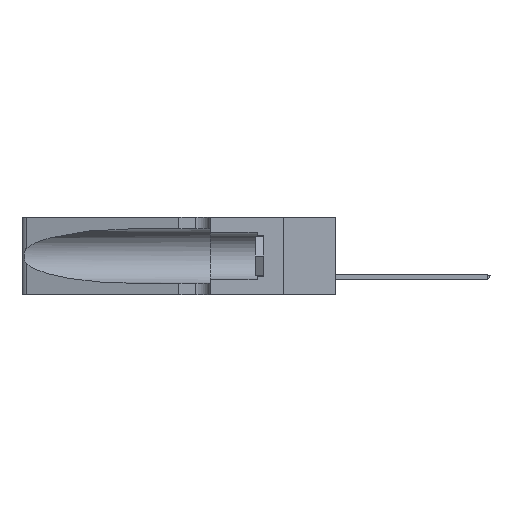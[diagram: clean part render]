
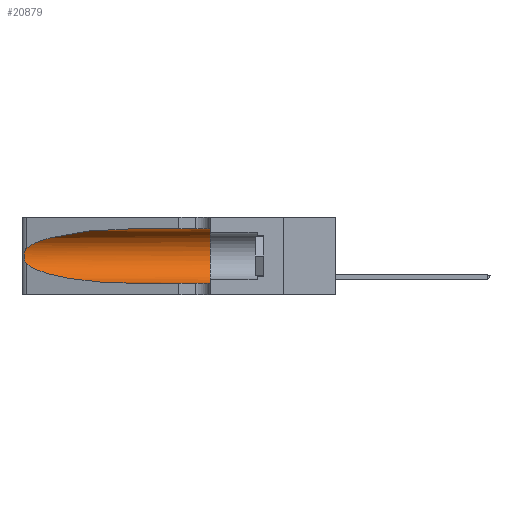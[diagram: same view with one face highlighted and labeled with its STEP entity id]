
A CAD part, left-side view. The second image highlights one B-rep face of the part: STEP entity #20879.
In plain terms, the highlighted cylindrical face has radius 3.308 mm (diameter 6.617 mm), a partial arc.
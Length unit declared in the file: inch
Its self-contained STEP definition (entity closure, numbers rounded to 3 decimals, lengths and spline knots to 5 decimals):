
#116 = B_SPLINE_CURVE_WITH_KNOTS ( 'NONE', 3,
 ( #9025, #15880, #19673, #1629, #12503, #10636, #21319, #10792, #19597, #17581, #23099, #5159, #19377, #5382 ),
 .UNSPECIFIED., .F., .F.,
 ( 4, 2, 2, 2, 2, 2, 4 ),
 ( 0., 0.00027, 0.00053, 0.00107, 0.0016, 0.00187, 0.00214 ),
 .UNSPECIFIED. ) ;
#762 = ORIENTED_EDGE ( 'NONE', *, *, #16962, .F. ) ;
#1184 = ORIENTED_EDGE ( 'NONE', *, *, #10674, .T. ) ;
#1629 = CARTESIAN_POINT ( 'NONE',  ( 0.25787, 1.23484, 0.2124 ) ) ;
#1871 = EDGE_CURVE ( 'NONE', #15046, #11909, #20135, .T. ) ;
#1888 = AXIS2_PLACEMENT_3D ( 'NONE', #19101, #22509, #6600 ) ;
#1976 = EDGE_CURVE ( 'NONE', #8461, #4619, #5324, .T. ) ;
#3780 = ORIENTED_EDGE ( 'NONE', *, *, #1871, .T. ) ;
#3968 = CARTESIAN_POINT ( 'NONE',  ( 0.18966, 0.96281, 0.31525 ) ) ;
#4028 = CYLINDRICAL_SURFACE ( 'NONE', #13454, 0.13025 ) ;
#4334 = LINE ( 'NONE', #12100, #22416 ) ;
#4619 = VERTEX_POINT ( 'NONE', #10180 ) ;
#5159 = CARTESIAN_POINT ( 'NONE',  ( 0.25639, 1.23186, 0.15144 ) ) ;
#5324 =( BOUNDED_CURVE ( )  B_SPLINE_CURVE ( 3, ( #9031, #3968, #19676, #19816 ),
 .UNSPECIFIED., .F., .T. ) 
 B_SPLINE_CURVE_WITH_KNOTS ( ( 4, 4 ),
 ( 1.5708, 2.84003 ),
 .UNSPECIFIED. ) 
 CURVE ( )  GEOMETRIC_REPRESENTATION_ITEM ( )  RATIONAL_B_SPLINE_CURVE ( ( 1., 0.87, 0.87, 1. ) ) 
 REPRESENTATION_ITEM ( '' )  );
#5382 = CARTESIAN_POINT ( 'NONE',  ( 0.25487, 1.22718, 0.14631 ) ) ;
#6600 = DIRECTION ( 'NONE',  ( 0., 0., 1. ) ) ;
#7967 = CIRCLE ( 'NONE', #1888, 0.13025 ) ;
#8461 = VERTEX_POINT ( 'NONE', #8618 ) ;
#8618 = CARTESIAN_POINT ( 'NONE',  ( 0.1305, 0.72297, 0.31525 ) ) ;
#8760 = FACE_OUTER_BOUND ( 'NONE', #20014, .T. ) ;
#8932 = CARTESIAN_POINT ( 'NONE',  ( 0.1305, 0.72297, 0.05475 ) ) ;
#9025 = CARTESIAN_POINT ( 'NONE',  ( 0.25487, 1.22718, 0.22369 ) ) ;
#9031 = CARTESIAN_POINT ( 'NONE',  ( 0.1305, 0.72297, 0.31525 ) ) ;
#9729 = DIRECTION ( 'NONE',  ( 0., -1., 0. ) ) ;
#10069 = ORIENTED_EDGE ( 'NONE', *, *, #19679, .F. ) ;
#10180 = CARTESIAN_POINT ( 'NONE',  ( 0.25487, 1.22718, 0.22369 ) ) ;
#10636 = CARTESIAN_POINT ( 'NONE',  ( 0.26018, 1.23835, 0.19895 ) ) ;
#10674 = EDGE_CURVE ( 'NONE', #11909, #17735, #15838, .T. ) ;
#10792 = CARTESIAN_POINT ( 'NONE',  ( 0.26075, 1.23896, 0.178 ) ) ;
#11480 = DIRECTION ( 'NONE',  ( 0., 0., -1. ) ) ;
#11909 = VERTEX_POINT ( 'NONE', #8932 ) ;
#12100 = CARTESIAN_POINT ( 'NONE',  ( 0.1305, 1.61858, 0.31525 ) ) ;
#12145 = CARTESIAN_POINT ( 'NONE',  ( 0.1305, 1.61858, 0.05475 ) ) ;
#12161 = ORIENTED_EDGE ( 'NONE', *, *, #13159, .T. ) ;
#12503 = CARTESIAN_POINT ( 'NONE',  ( 0.25854, 1.2359, 0.20912 ) ) ;
#13159 = EDGE_CURVE ( 'NONE', #4619, #15046, #116, .T. ) ;
#13454 = AXIS2_PLACEMENT_3D ( 'NONE', #15027, #9729, #11480 ) ;
#14112 = CARTESIAN_POINT ( 'NONE',  ( 0.25487, 1.22718, 0.14631 ) ) ;
#14840 = CARTESIAN_POINT ( 'NONE',  ( 0.25487, 1.22718, 0.14631 ) ) ;
#15011 = CARTESIAN_POINT ( 'NONE',  ( 0.1305, 0.35, 0.05475 ) ) ;
#15027 = CARTESIAN_POINT ( 'NONE',  ( 0.1305, 1.61858, 0.185 ) ) ;
#15046 = VERTEX_POINT ( 'NONE', #14112 ) ;
#15838 = LINE ( 'NONE', #12145, #20541 ) ;
#15852 = DIRECTION ( 'NONE',  ( 0., -1., 0. ) ) ;
#15880 = CARTESIAN_POINT ( 'NONE',  ( 0.25555, 1.22994, 0.2215 ) ) ;
#16962 = EDGE_CURVE ( 'NONE', #19148, #17735, #7967, .T. ) ;
#17161 = CARTESIAN_POINT ( 'NONE',  ( 0.2373, 1.15595, 0.08982 ) ) ;
#17473 = CARTESIAN_POINT ( 'NONE',  ( 0.1305, 0.72297, 0.05475 ) ) ;
#17581 = CARTESIAN_POINT ( 'NONE',  ( 0.25856, 1.23593, 0.16098 ) ) ;
#17735 = VERTEX_POINT ( 'NONE', #15011 ) ;
#19101 = CARTESIAN_POINT ( 'NONE',  ( 0.1305, 0.35, 0.185 ) ) ;
#19148 = VERTEX_POINT ( 'NONE', #19623 ) ;
#19377 = CARTESIAN_POINT ( 'NONE',  ( 0.25555, 1.22993, 0.14849 ) ) ;
#19597 = CARTESIAN_POINT ( 'NONE',  ( 0.26017, 1.23833, 0.17102 ) ) ;
#19623 = CARTESIAN_POINT ( 'NONE',  ( 0.1305, 0.35, 0.31525 ) ) ;
#19673 = CARTESIAN_POINT ( 'NONE',  ( 0.25639, 1.23184, 0.21858 ) ) ;
#19676 = CARTESIAN_POINT ( 'NONE',  ( 0.2373, 1.15595, 0.28018 ) ) ;
#19679 = EDGE_CURVE ( 'NONE', #8461, #19148, #4334, .T. ) ;
#19816 = CARTESIAN_POINT ( 'NONE',  ( 0.25487, 1.22718, 0.22369 ) ) ;
#20014 = EDGE_LOOP ( 'NONE', ( #22793, #12161, #3780, #1184, #762, #10069 ) ) ;
#20135 =( BOUNDED_CURVE ( )  B_SPLINE_CURVE ( 3, ( #14840, #17161, #21056, #17473 ),
 .UNSPECIFIED., .F., .F. ) 
 B_SPLINE_CURVE_WITH_KNOTS ( ( 4, 4 ),
 ( 3.44316, 4.71239 ),
 .UNSPECIFIED. ) 
 CURVE ( )  GEOMETRIC_REPRESENTATION_ITEM ( )  RATIONAL_B_SPLINE_CURVE ( ( 1., 0.87, 0.87, 1. ) ) 
 REPRESENTATION_ITEM ( '' )  );
#20541 = VECTOR ( 'NONE', #15852, 39.37008 ) ;
#20879 = ADVANCED_FACE ( 'NONE', ( #8760 ), #4028, .F. ) ;
#21056 = CARTESIAN_POINT ( 'NONE',  ( 0.18966, 0.96281, 0.05475 ) ) ;
#21319 = CARTESIAN_POINT ( 'NONE',  ( 0.26075, 1.23896, 0.19203 ) ) ;
#22416 = VECTOR ( 'NONE', #22943, 39.37008 ) ;
#22509 = DIRECTION ( 'NONE',  ( 0., 1., 0. ) ) ;
#22793 = ORIENTED_EDGE ( 'NONE', *, *, #1976, .T. ) ;
#22943 = DIRECTION ( 'NONE',  ( 0., -1., 0. ) ) ;
#23099 = CARTESIAN_POINT ( 'NONE',  ( 0.25789, 1.23486, 0.15765 ) ) ;
